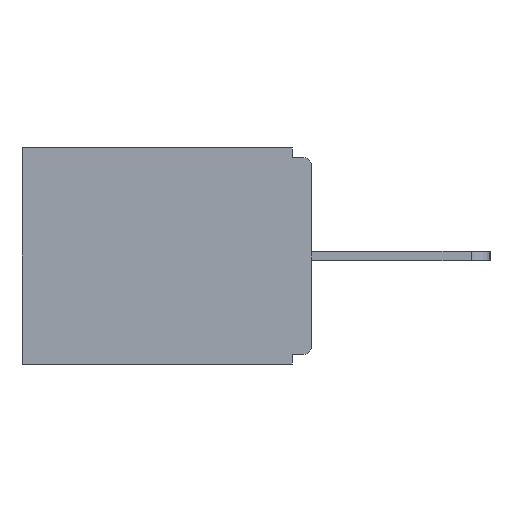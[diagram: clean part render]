
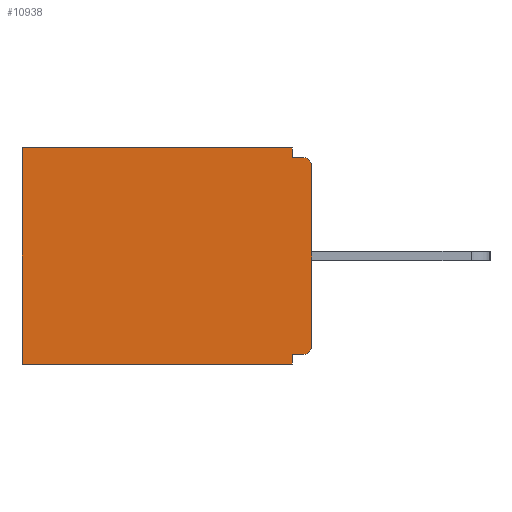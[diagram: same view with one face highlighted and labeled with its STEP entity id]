
A CAD part, left-side view. The second image highlights one B-rep face of the part: STEP entity #10938.
In plain terms, the highlighted planar face has unit normal (-1, 0, 0).
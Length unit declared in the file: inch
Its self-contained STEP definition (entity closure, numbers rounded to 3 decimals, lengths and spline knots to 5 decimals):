
#29 = DIRECTION ( 'NONE',  ( 0., -1., 0. ) ) ;
#82 = VECTOR ( 'NONE', #25922, 39.37008 ) ;
#333 = VERTEX_POINT ( 'NONE', #3552 ) ;
#360 = EDGE_CURVE ( 'NONE', #5038, #5680, #12556, .T. ) ;
#693 = EDGE_LOOP ( 'NONE', ( #20122, #4401, #7757, #2107, #10811, #5889, #20479, #6039, #24601, #24355 ) ) ;
#771 = CARTESIAN_POINT ( 'NONE',  ( 0.298, 0.46, -0.343 ) ) ;
#990 = VECTOR ( 'NONE', #24286, 39.37008 ) ;
#1252 = LINE ( 'NONE', #19407, #2523 ) ;
#1709 = CIRCLE ( 'NONE', #10025, 0.015 ) ;
#1781 = DIRECTION ( 'NONE',  ( 0., 0., -1. ) ) ;
#2107 = ORIENTED_EDGE ( 'NONE', *, *, #2422, .T. ) ;
#2422 = EDGE_CURVE ( 'NONE', #6421, #333, #24154, .T. ) ;
#2523 = VECTOR ( 'NONE', #21580, 39.37008 ) ;
#2605 = CARTESIAN_POINT ( 'NONE',  ( 0.298, 0.031, -0.343 ) ) ;
#2683 = EDGE_CURVE ( 'NONE', #12701, #5680, #1709, .T. ) ;
#3036 = DIRECTION ( 'NONE',  ( 0., 0., -1. ) ) ;
#3552 = CARTESIAN_POINT ( 'NONE',  ( 0.298, 0.46, 0. ) ) ;
#4401 = ORIENTED_EDGE ( 'NONE', *, *, #360, .F. ) ;
#5038 = VERTEX_POINT ( 'NONE', #9829 ) ;
#5067 = LINE ( 'NONE', #6366, #12963 ) ;
#5680 = VERTEX_POINT ( 'NONE', #13917 ) ;
#5834 = CARTESIAN_POINT ( 'NONE',  ( 0.298, 0., -0.328 ) ) ;
#5889 = ORIENTED_EDGE ( 'NONE', *, *, #7678, .F. ) ;
#6039 = ORIENTED_EDGE ( 'NONE', *, *, #23506, .F. ) ;
#6239 = AXIS2_PLACEMENT_3D ( 'NONE', #22456, #18545, #10318 ) ;
#6366 = CARTESIAN_POINT ( 'NONE',  ( 0.298, 0.46, 0. ) ) ;
#6421 = VERTEX_POINT ( 'NONE', #25919 ) ;
#6513 = EDGE_CURVE ( 'NONE', #19994, #19873, #8920, .T. ) ;
#6916 = DIRECTION ( 'NONE',  ( 0., 1., 0. ) ) ;
#7678 = EDGE_CURVE ( 'NONE', #25214, #25997, #18382, .T. ) ;
#7757 = ORIENTED_EDGE ( 'NONE', *, *, #12270, .F. ) ;
#7793 = EDGE_CURVE ( 'NONE', #333, #25997, #5067, .T. ) ;
#8150 = AXIS2_PLACEMENT_3D ( 'NONE', #15829, #9876, #9781 ) ;
#8920 = CIRCLE ( 'NONE', #6239, 0.015 ) ;
#9781 = DIRECTION ( 'NONE',  ( 0., 0., -1. ) ) ;
#9829 = CARTESIAN_POINT ( 'NONE',  ( 0.298, 0.031, -0.015 ) ) ;
#9876 = DIRECTION ( 'NONE',  ( 1., 0., 0. ) ) ;
#10025 = AXIS2_PLACEMENT_3D ( 'NONE', #23940, #11854, #1781 ) ;
#10055 = DIRECTION ( 'NONE',  ( 0., 0., -1. ) ) ;
#10318 = DIRECTION ( 'NONE',  ( 0., 0., -1. ) ) ;
#10811 = ORIENTED_EDGE ( 'NONE', *, *, #7793, .T. ) ;
#10938 = ADVANCED_FACE ( 'NONE', ( #24571 ), #17762, .F. ) ;
#11674 = VECTOR ( 'NONE', #3036, 39.37008 ) ;
#11851 = CARTESIAN_POINT ( 'NONE',  ( 0.298, 0., -0.343 ) ) ;
#11854 = DIRECTION ( 'NONE',  ( -1., 0., 0. ) ) ;
#12270 = EDGE_CURVE ( 'NONE', #6421, #5038, #23695, .T. ) ;
#12273 = VECTOR ( 'NONE', #14987, 39.37008 ) ;
#12556 = LINE ( 'NONE', #18282, #18273 ) ;
#12701 = VERTEX_POINT ( 'NONE', #13131 ) ;
#12735 = EDGE_CURVE ( 'NONE', #19727, #25214, #1252, .T. ) ;
#12902 = LINE ( 'NONE', #16871, #12273 ) ;
#12963 = VECTOR ( 'NONE', #10055, 39.37008 ) ;
#12985 = CARTESIAN_POINT ( 'NONE',  ( 0.298, 0., -0.313 ) ) ;
#13131 = CARTESIAN_POINT ( 'NONE',  ( 0.298, 0., -0.03 ) ) ;
#13917 = CARTESIAN_POINT ( 'NONE',  ( 0.298, 0.015, -0.015 ) ) ;
#14987 = DIRECTION ( 'NONE',  ( 0., 0., -1. ) ) ;
#15829 = CARTESIAN_POINT ( 'NONE',  ( 0.298, 0., 0. ) ) ;
#16871 = CARTESIAN_POINT ( 'NONE',  ( 0.298, 0., 0. ) ) ;
#17177 = CARTESIAN_POINT ( 'NONE',  ( 0.298, 0.015, -0.328 ) ) ;
#17762 = PLANE ( 'NONE',  #8150 ) ;
#18273 = VECTOR ( 'NONE', #29, 39.37008 ) ;
#18282 = CARTESIAN_POINT ( 'NONE',  ( 0.298, 0., -0.015 ) ) ;
#18382 = LINE ( 'NONE', #11851, #82 ) ;
#18545 = DIRECTION ( 'NONE',  ( -1., 0., 0. ) ) ;
#18685 = LINE ( 'NONE', #5834, #990 ) ;
#19407 = CARTESIAN_POINT ( 'NONE',  ( 0.298, 0.031, -0.343 ) ) ;
#19727 = VERTEX_POINT ( 'NONE', #20525 ) ;
#19873 = VERTEX_POINT ( 'NONE', #12985 ) ;
#19994 = VERTEX_POINT ( 'NONE', #17177 ) ;
#20122 = ORIENTED_EDGE ( 'NONE', *, *, #2683, .T. ) ;
#20479 = ORIENTED_EDGE ( 'NONE', *, *, #12735, .F. ) ;
#20525 = CARTESIAN_POINT ( 'NONE',  ( 0.298, 0.031, -0.328 ) ) ;
#21580 = DIRECTION ( 'NONE',  ( 0., 0., -1. ) ) ;
#22285 = VECTOR ( 'NONE', #6916, 39.37008 ) ;
#22456 = CARTESIAN_POINT ( 'NONE',  ( 0.298, 0.015, -0.313 ) ) ;
#22902 = CARTESIAN_POINT ( 'NONE',  ( 0.298, 0., 0. ) ) ;
#23343 = CARTESIAN_POINT ( 'NONE',  ( 0.298, 0.031, -0.343 ) ) ;
#23506 = EDGE_CURVE ( 'NONE', #19994, #19727, #18685, .T. ) ;
#23695 = LINE ( 'NONE', #23343, #11674 ) ;
#23940 = CARTESIAN_POINT ( 'NONE',  ( 0.298, 0.015, -0.03 ) ) ;
#24154 = LINE ( 'NONE', #22902, #22285 ) ;
#24286 = DIRECTION ( 'NONE',  ( 0., 1., 0. ) ) ;
#24355 = ORIENTED_EDGE ( 'NONE', *, *, #24705, .F. ) ;
#24571 = FACE_OUTER_BOUND ( 'NONE', #693, .T. ) ;
#24601 = ORIENTED_EDGE ( 'NONE', *, *, #6513, .T. ) ;
#24705 = EDGE_CURVE ( 'NONE', #12701, #19873, #12902, .T. ) ;
#25214 = VERTEX_POINT ( 'NONE', #2605 ) ;
#25919 = CARTESIAN_POINT ( 'NONE',  ( 0.298, 0.031, 0. ) ) ;
#25922 = DIRECTION ( 'NONE',  ( 0., 1., 0. ) ) ;
#25997 = VERTEX_POINT ( 'NONE', #771 ) ;
